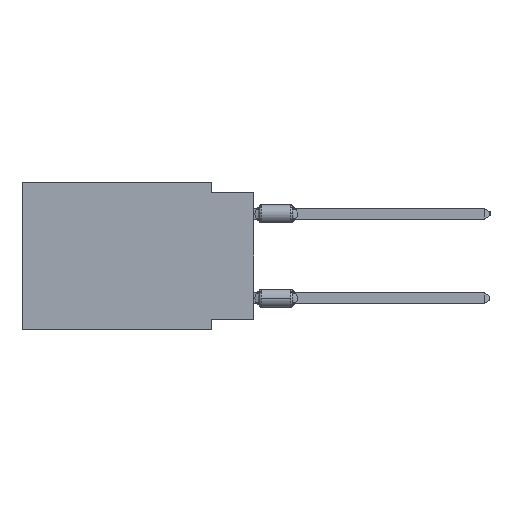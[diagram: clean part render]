
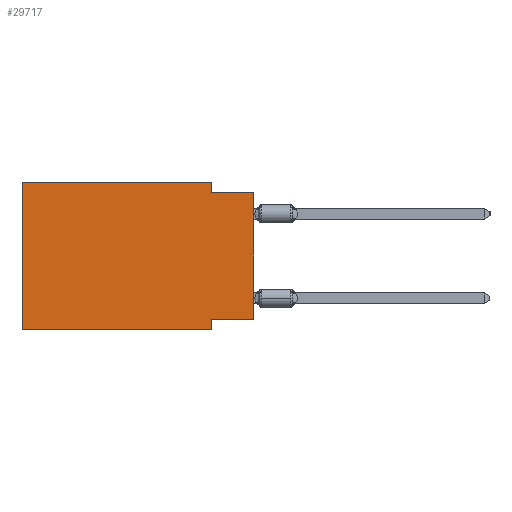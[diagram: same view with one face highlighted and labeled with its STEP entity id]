
A CAD part, left-side view. The second image highlights one B-rep face of the part: STEP entity #29717.
In plain terms, the highlighted planar face has unit normal (-1, 0, 0).
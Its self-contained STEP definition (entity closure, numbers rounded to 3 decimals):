
#1951 = AXIS2_PLACEMENT_3D ( 'NONE', #17718, #26354, #24324 ) ;
#2217 = EDGE_CURVE ( 'NONE', #27959, #34562, #34938, .T. ) ;
#3204 = CARTESIAN_POINT ( 'NONE',  ( 0., 0., -0.635 ) ) ;
#3764 = VERTEX_POINT ( 'NONE', #27547 ) ;
#4412 = CARTESIAN_POINT ( 'NONE',  ( 0., 0., -8.255 ) ) ;
#4542 = DIRECTION ( 'NONE',  ( 0., 1., 0. ) ) ;
#4807 = VECTOR ( 'NONE', #9808, 1000. ) ;
#4900 = DIRECTION ( 'NONE',  ( 0., -1., 0. ) ) ;
#5626 = CARTESIAN_POINT ( 'NONE',  ( 0., 2.54, -8.89 ) ) ;
#6814 = EDGE_CURVE ( 'NONE', #38190, #20303, #31490, .T. ) ;
#6824 = VECTOR ( 'NONE', #17611, 1000. ) ;
#7410 = DIRECTION ( 'NONE',  ( 0., 0., 1. ) ) ;
#7453 = CARTESIAN_POINT ( 'NONE',  ( 0., 13.97, 0. ) ) ;
#8209 = CARTESIAN_POINT ( 'NONE',  ( 0., 0., -0.635 ) ) ;
#9808 = DIRECTION ( 'NONE',  ( 0., 0., 1. ) ) ;
#11556 = LINE ( 'NONE', #26296, #24347 ) ;
#11637 = VERTEX_POINT ( 'NONE', #20280 ) ;
#12108 = ORIENTED_EDGE ( 'NONE', *, *, #6814, .F. ) ;
#12623 = ORIENTED_EDGE ( 'NONE', *, *, #27256, .F. ) ;
#13943 = CARTESIAN_POINT ( 'NONE',  ( 0., 2.54, 0. ) ) ;
#15394 = EDGE_CURVE ( 'NONE', #20303, #3764, #18192, .T. ) ;
#16508 = LINE ( 'NONE', #34395, #33373 ) ;
#16677 = LINE ( 'NONE', #7453, #4807 ) ;
#17611 = DIRECTION ( 'NONE',  ( 0., 0., -1. ) ) ;
#17718 = CARTESIAN_POINT ( 'NONE',  ( 0., 13.97, 0. ) ) ;
#18192 = LINE ( 'NONE', #5626, #6824 ) ;
#18501 = ORIENTED_EDGE ( 'NONE', *, *, #2217, .F. ) ;
#18737 = ORIENTED_EDGE ( 'NONE', *, *, #31425, .F. ) ;
#19502 = VECTOR ( 'NONE', #23330, 1000. ) ;
#20279 = PLANE ( 'NONE',  #1951 ) ;
#20280 = CARTESIAN_POINT ( 'NONE',  ( 0., 13.97, 0. ) ) ;
#20303 = VERTEX_POINT ( 'NONE', #24694 ) ;
#21248 = ORIENTED_EDGE ( 'NONE', *, *, #24556, .F. ) ;
#21517 = EDGE_CURVE ( 'NONE', #38190, #34562, #25287, .T. ) ;
#21775 = CARTESIAN_POINT ( 'NONE',  ( 0., 13.97, -8.89 ) ) ;
#22141 = CARTESIAN_POINT ( 'NONE',  ( 0., 0., 0. ) ) ;
#22594 = CARTESIAN_POINT ( 'NONE',  ( 0., 0., -8.255 ) ) ;
#23330 = DIRECTION ( 'NONE',  ( 0., -1., 0. ) ) ;
#24074 = VECTOR ( 'NONE', #7410, 1000. ) ;
#24324 = DIRECTION ( 'NONE',  ( 0., 0., -1. ) ) ;
#24347 = VECTOR ( 'NONE', #30045, 1000. ) ;
#24556 = EDGE_CURVE ( 'NONE', #29553, #11637, #16677, .T. ) ;
#24694 = CARTESIAN_POINT ( 'NONE',  ( 0., 2.54, -8.255 ) ) ;
#24731 = LINE ( 'NONE', #21775, #28684 ) ;
#25287 = LINE ( 'NONE', #22141, #24074 ) ;
#26296 = CARTESIAN_POINT ( 'NONE',  ( 0., 2.54, 0. ) ) ;
#26354 = DIRECTION ( 'NONE',  ( 1., 0., 0. ) ) ;
#26709 = ORIENTED_EDGE ( 'NONE', *, *, #21517, .T. ) ;
#27256 = EDGE_CURVE ( 'NONE', #32656, #27959, #11556, .T. ) ;
#27547 = CARTESIAN_POINT ( 'NONE',  ( 0., 2.54, -8.89 ) ) ;
#27959 = VERTEX_POINT ( 'NONE', #28543 ) ;
#28543 = CARTESIAN_POINT ( 'NONE',  ( 0., 2.54, -0.635 ) ) ;
#28684 = VECTOR ( 'NONE', #38290, 1000. ) ;
#29047 = VECTOR ( 'NONE', #4542, 1000. ) ;
#29553 = VERTEX_POINT ( 'NONE', #37008 ) ;
#29717 = ADVANCED_FACE ( 'NONE', ( #38362 ), #20279, .F. ) ;
#29875 = ORIENTED_EDGE ( 'NONE', *, *, #15394, .F. ) ;
#30045 = DIRECTION ( 'NONE',  ( 0., 0., -1. ) ) ;
#31425 = EDGE_CURVE ( 'NONE', #11637, #32656, #16508, .T. ) ;
#31490 = LINE ( 'NONE', #22594, #29047 ) ;
#32656 = VERTEX_POINT ( 'NONE', #13943 ) ;
#33373 = VECTOR ( 'NONE', #4900, 1000. ) ;
#34395 = CARTESIAN_POINT ( 'NONE',  ( 0., 13.97, 0. ) ) ;
#34562 = VERTEX_POINT ( 'NONE', #3204 ) ;
#34938 = LINE ( 'NONE', #8209, #19502 ) ;
#36300 = EDGE_CURVE ( 'NONE', #29553, #3764, #24731, .T. ) ;
#37008 = CARTESIAN_POINT ( 'NONE',  ( 0., 13.97, -8.89 ) ) ;
#37090 = ORIENTED_EDGE ( 'NONE', *, *, #36300, .T. ) ;
#37411 = EDGE_LOOP ( 'NONE', ( #26709, #18501, #12623, #18737, #21248, #37090, #29875, #12108 ) ) ;
#38190 = VERTEX_POINT ( 'NONE', #4412 ) ;
#38290 = DIRECTION ( 'NONE',  ( 0., -1., 0. ) ) ;
#38362 = FACE_OUTER_BOUND ( 'NONE', #37411, .T. ) ;
